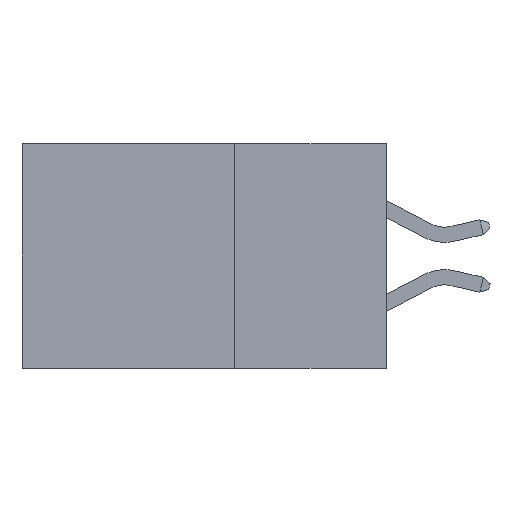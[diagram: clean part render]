
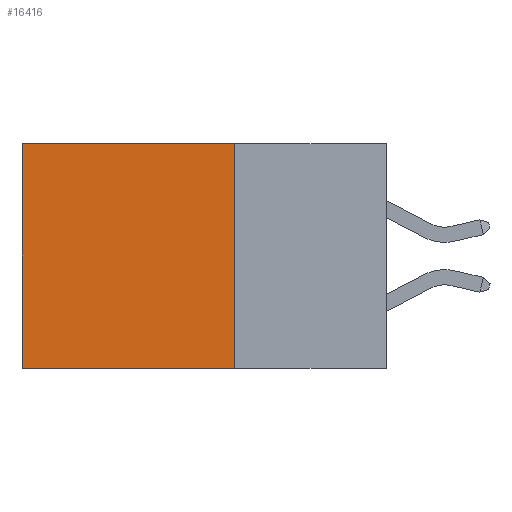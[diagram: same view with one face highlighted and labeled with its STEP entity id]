
A CAD part, left-side view. The second image highlights one B-rep face of the part: STEP entity #16416.
In plain terms, the highlighted planar face has unit normal (-1, 0, 0).
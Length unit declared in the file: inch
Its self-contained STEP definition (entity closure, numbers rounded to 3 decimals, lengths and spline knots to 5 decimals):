
#34 = LINE ( 'NONE', #19336, #21481 ) ;
#526 = PLANE ( 'NONE',  #12237 ) ;
#1331 = DIRECTION ( 'NONE',  ( 0., 1., 0. ) ) ;
#2939 = LINE ( 'NONE', #20043, #23161 ) ;
#3050 = VERTEX_POINT ( 'NONE', #14456 ) ;
#3929 = CARTESIAN_POINT ( 'NONE',  ( 0.298, 0.6, 0. ) ) ;
#4448 = CARTESIAN_POINT ( 'NONE',  ( 0.298, 0.25, 0. ) ) ;
#5233 = EDGE_CURVE ( 'NONE', #10580, #8543, #7340, .T. ) ;
#7340 = LINE ( 'NONE', #16681, #18583 ) ;
#8361 = DIRECTION ( 'NONE',  ( 1., 0., 0. ) ) ;
#8543 = VERTEX_POINT ( 'NONE', #9839 ) ;
#9839 = CARTESIAN_POINT ( 'NONE',  ( 0.298, 0.25, -0.37 ) ) ;
#10446 = DIRECTION ( 'NONE',  ( 0., 0., -1. ) ) ;
#10580 = VERTEX_POINT ( 'NONE', #16616 ) ;
#11956 = EDGE_CURVE ( 'NONE', #14955, #3050, #22257, .T. ) ;
#12047 = DIRECTION ( 'NONE',  ( 0., 1., 0. ) ) ;
#12237 = AXIS2_PLACEMENT_3D ( 'NONE', #4448, #8361, #10446 ) ;
#13317 = ORIENTED_EDGE ( 'NONE', *, *, #14462, .T. ) ;
#13417 = EDGE_LOOP ( 'NONE', ( #16127, #22903, #23777, #13317 ) ) ;
#14456 = CARTESIAN_POINT ( 'NONE',  ( 0.298, 0.6, -0.37 ) ) ;
#14462 = EDGE_CURVE ( 'NONE', #10580, #14955, #34, .T. ) ;
#14955 = VERTEX_POINT ( 'NONE', #25004 ) ;
#16127 = ORIENTED_EDGE ( 'NONE', *, *, #11956, .T. ) ;
#16416 = ADVANCED_FACE ( 'NONE', ( #25094 ), #526, .F. ) ;
#16616 = CARTESIAN_POINT ( 'NONE',  ( 0.298, 0.25, 0. ) ) ;
#16681 = CARTESIAN_POINT ( 'NONE',  ( 0.298, 0.25, 0. ) ) ;
#18583 = VECTOR ( 'NONE', #22646, 39.37008 ) ;
#19336 = CARTESIAN_POINT ( 'NONE',  ( 0.298, 0.25, 0. ) ) ;
#19790 = VECTOR ( 'NONE', #23731, 39.37008 ) ;
#20043 = CARTESIAN_POINT ( 'NONE',  ( 0.298, 0.25, -0.37 ) ) ;
#21481 = VECTOR ( 'NONE', #1331, 39.37008 ) ;
#21842 = EDGE_CURVE ( 'NONE', #8543, #3050, #2939, .T. ) ;
#22257 = LINE ( 'NONE', #3929, #19790 ) ;
#22646 = DIRECTION ( 'NONE',  ( 0., 0., -1. ) ) ;
#22903 = ORIENTED_EDGE ( 'NONE', *, *, #21842, .F. ) ;
#23161 = VECTOR ( 'NONE', #12047, 39.37008 ) ;
#23731 = DIRECTION ( 'NONE',  ( 0., 0., -1. ) ) ;
#23777 = ORIENTED_EDGE ( 'NONE', *, *, #5233, .F. ) ;
#25004 = CARTESIAN_POINT ( 'NONE',  ( 0.298, 0.6, 0. ) ) ;
#25094 = FACE_OUTER_BOUND ( 'NONE', #13417, .T. ) ;
